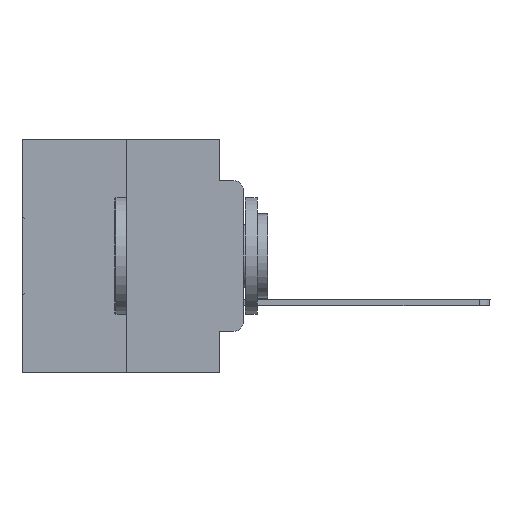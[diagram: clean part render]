
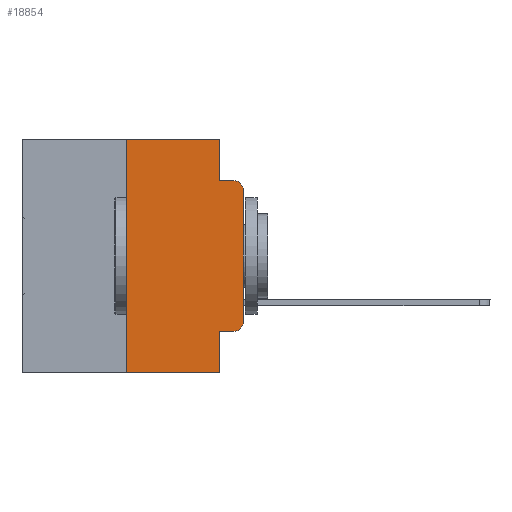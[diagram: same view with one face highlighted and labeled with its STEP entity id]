
A CAD part, left-side view. The second image highlights one B-rep face of the part: STEP entity #18854.
In plain terms, the highlighted planar face has unit normal (-1, 0, 0).
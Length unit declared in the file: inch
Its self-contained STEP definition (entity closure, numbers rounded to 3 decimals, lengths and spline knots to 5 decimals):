
#428 = ORIENTED_EDGE ( 'NONE', *, *, #17525, .T. ) ;
#708 = CARTESIAN_POINT ( 'NONE',  ( 0., 0.25, -0.5 ) ) ;
#1581 = LINE ( 'NONE', #10919, #30847 ) ;
#1748 = CARTESIAN_POINT ( 'NONE',  ( 0., 0.473, 0. ) ) ;
#1810 = VECTOR ( 'NONE', #28640, 39.37008 ) ;
#1954 = LINE ( 'NONE', #23704, #3075 ) ;
#2037 = VECTOR ( 'NONE', #5085, 39.37008 ) ;
#2226 = ORIENTED_EDGE ( 'NONE', *, *, #14119, .F. ) ;
#2391 = DIRECTION ( 'NONE',  ( 0., 0., -1. ) ) ;
#3045 = CIRCLE ( 'NONE', #7571, 0.02 ) ;
#3075 = VECTOR ( 'NONE', #23544, 39.37008 ) ;
#3446 = CARTESIAN_POINT ( 'NONE',  ( 0., 0.02, -0.1085 ) ) ;
#4119 = EDGE_CURVE ( 'NONE', #11070, #17460, #4410, .T. ) ;
#4410 = LINE ( 'NONE', #23923, #6957 ) ;
#4840 = VECTOR ( 'NONE', #11925, 39.37008 ) ;
#4867 = AXIS2_PLACEMENT_3D ( 'NONE', #4909, #19254, #14215 ) ;
#4909 = CARTESIAN_POINT ( 'NONE',  ( 0., 0.02, -0.3915 ) ) ;
#5085 = DIRECTION ( 'NONE',  ( 0., -1., 0. ) ) ;
#6136 = CARTESIAN_POINT ( 'NONE',  ( 0., 0.02, -0.4115 ) ) ;
#6200 = CARTESIAN_POINT ( 'NONE',  ( 0., 0.051, 0. ) ) ;
#6304 = CARTESIAN_POINT ( 'NONE',  ( 0., 0.051, -0.5 ) ) ;
#6309 = AXIS2_PLACEMENT_3D ( 'NONE', #1748, #11861, #2391 ) ;
#6885 = CARTESIAN_POINT ( 'NONE',  ( 0., 0.051, -0.0885 ) ) ;
#6957 = VECTOR ( 'NONE', #11658, 39.37008 ) ;
#6984 = EDGE_LOOP ( 'NONE', ( #428, #15785, #30109, #14829, #26774, #20353, #20043, #2226, #9598, #27590 ) ) ;
#7125 = VERTEX_POINT ( 'NONE', #6304 ) ;
#7571 = AXIS2_PLACEMENT_3D ( 'NONE', #3446, #14807, #27231 ) ;
#7727 = EDGE_CURVE ( 'NONE', #17460, #29681, #14619, .T. ) ;
#7929 = EDGE_CURVE ( 'NONE', #12704, #24613, #14017, .T. ) ;
#8571 = VERTEX_POINT ( 'NONE', #19171 ) ;
#9138 = DIRECTION ( 'NONE',  ( 0., 0., -1. ) ) ;
#9265 = CARTESIAN_POINT ( 'NONE',  ( 0., 0.473, 0. ) ) ;
#9598 = ORIENTED_EDGE ( 'NONE', *, *, #7929, .T. ) ;
#9647 = FACE_OUTER_BOUND ( 'NONE', #6984, .T. ) ;
#10068 = VERTEX_POINT ( 'NONE', #20861 ) ;
#10752 = CARTESIAN_POINT ( 'NONE',  ( 0., 0.051, -0.0885 ) ) ;
#10919 = CARTESIAN_POINT ( 'NONE',  ( 0., 0., 0. ) ) ;
#11070 = VERTEX_POINT ( 'NONE', #708 ) ;
#11658 = DIRECTION ( 'NONE',  ( 0., 0., 1. ) ) ;
#11861 = DIRECTION ( 'NONE',  ( 1., 0., 0. ) ) ;
#11925 = DIRECTION ( 'NONE',  ( 0., -1., 0. ) ) ;
#12704 = VERTEX_POINT ( 'NONE', #20712 ) ;
#13411 = EDGE_CURVE ( 'NONE', #23211, #8571, #3045, .T. ) ;
#14017 = LINE ( 'NONE', #30871, #1810 ) ;
#14119 = EDGE_CURVE ( 'NONE', #12704, #7125, #1954, .T. ) ;
#14215 = DIRECTION ( 'NONE',  ( 0., 0., -1. ) ) ;
#14268 = CARTESIAN_POINT ( 'NONE',  ( 0., 0., -0.1085 ) ) ;
#14619 = LINE ( 'NONE', #9265, #29977 ) ;
#14807 = DIRECTION ( 'NONE',  ( -1., 0., 0. ) ) ;
#14821 = VERTEX_POINT ( 'NONE', #10752 ) ;
#14829 = ORIENTED_EDGE ( 'NONE', *, *, #28418, .F. ) ;
#15346 = DIRECTION ( 'NONE',  ( 0., 0., 1. ) ) ;
#15785 = ORIENTED_EDGE ( 'NONE', *, *, #13411, .T. ) ;
#17069 = CARTESIAN_POINT ( 'NONE',  ( 0., 0.473, -0.5 ) ) ;
#17460 = VERTEX_POINT ( 'NONE', #22567 ) ;
#17525 = EDGE_CURVE ( 'NONE', #10068, #23211, #1581, .T. ) ;
#18854 = ADVANCED_FACE ( 'NONE', ( #9647 ), #28539, .F. ) ;
#19171 = CARTESIAN_POINT ( 'NONE',  ( 0., 0.02, -0.0885 ) ) ;
#19254 = DIRECTION ( 'NONE',  ( -1., 0., 0. ) ) ;
#20043 = ORIENTED_EDGE ( 'NONE', *, *, #25676, .T. ) ;
#20353 = ORIENTED_EDGE ( 'NONE', *, *, #4119, .F. ) ;
#20603 = EDGE_CURVE ( 'NONE', #24613, #10068, #27995, .T. ) ;
#20712 = CARTESIAN_POINT ( 'NONE',  ( 0., 0.051, -0.4115 ) ) ;
#20861 = CARTESIAN_POINT ( 'NONE',  ( 0., 0., -0.3915 ) ) ;
#21429 = EDGE_CURVE ( 'NONE', #14821, #8571, #26076, .T. ) ;
#22567 = CARTESIAN_POINT ( 'NONE',  ( 0., 0.25, 0. ) ) ;
#23211 = VERTEX_POINT ( 'NONE', #14268 ) ;
#23544 = DIRECTION ( 'NONE',  ( 0., 0., -1. ) ) ;
#23704 = CARTESIAN_POINT ( 'NONE',  ( 0., 0.051, 0. ) ) ;
#23923 = CARTESIAN_POINT ( 'NONE',  ( 0., 0.25, 0. ) ) ;
#24214 = DIRECTION ( 'NONE',  ( 0., -1., 0. ) ) ;
#24613 = VERTEX_POINT ( 'NONE', #6136 ) ;
#25676 = EDGE_CURVE ( 'NONE', #11070, #7125, #29341, .T. ) ;
#26076 = LINE ( 'NONE', #6885, #4840 ) ;
#26774 = ORIENTED_EDGE ( 'NONE', *, *, #7727, .F. ) ;
#27231 = DIRECTION ( 'NONE',  ( 0., 0., -1. ) ) ;
#27590 = ORIENTED_EDGE ( 'NONE', *, *, #20603, .T. ) ;
#27761 = VECTOR ( 'NONE', #9138, 39.37008 ) ;
#27995 = CIRCLE ( 'NONE', #4867, 0.02 ) ;
#28184 = CARTESIAN_POINT ( 'NONE',  ( 0., 0.051, 0. ) ) ;
#28418 = EDGE_CURVE ( 'NONE', #29681, #14821, #28652, .T. ) ;
#28539 = PLANE ( 'NONE',  #6309 ) ;
#28640 = DIRECTION ( 'NONE',  ( 0., -1., 0. ) ) ;
#28652 = LINE ( 'NONE', #28184, #27761 ) ;
#29341 = LINE ( 'NONE', #17069, #2037 ) ;
#29681 = VERTEX_POINT ( 'NONE', #6200 ) ;
#29977 = VECTOR ( 'NONE', #24214, 39.37008 ) ;
#30109 = ORIENTED_EDGE ( 'NONE', *, *, #21429, .F. ) ;
#30847 = VECTOR ( 'NONE', #15346, 39.37008 ) ;
#30871 = CARTESIAN_POINT ( 'NONE',  ( 0., 0.051, -0.4115 ) ) ;
